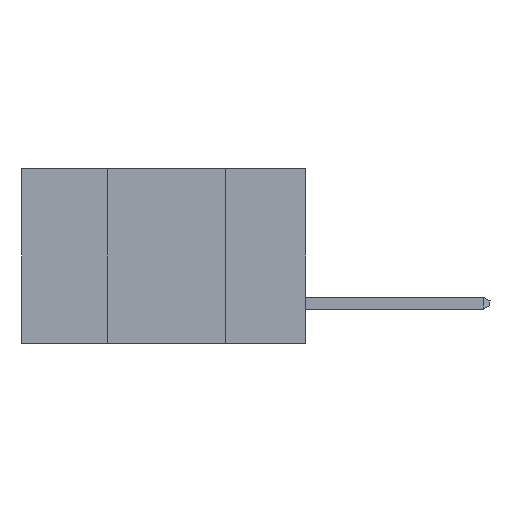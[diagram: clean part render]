
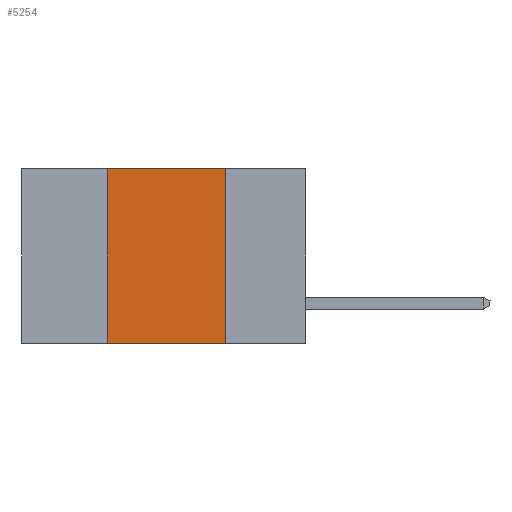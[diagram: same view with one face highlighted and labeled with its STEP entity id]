
A CAD part, left-side view. The second image highlights one B-rep face of the part: STEP entity #5254.
In plain terms, the highlighted planar face has unit normal (-1, 0, 0).
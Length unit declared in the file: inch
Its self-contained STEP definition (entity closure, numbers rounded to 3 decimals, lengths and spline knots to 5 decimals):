
#1218 = CARTESIAN_POINT ( 'NONE',  ( 0., 0.42, -0.37 ) ) ;
#2093 = ORIENTED_EDGE ( 'NONE', *, *, #2721, .F. ) ;
#2637 = CARTESIAN_POINT ( 'NONE',  ( 0., 0.17, -0.37 ) ) ;
#2721 = EDGE_CURVE ( 'NONE', #3608, #12944, #9174, .T. ) ;
#2815 = CARTESIAN_POINT ( 'NONE',  ( 0., 0.42, -0.37 ) ) ;
#2840 = VECTOR ( 'NONE', #8905, 39.37008 ) ;
#3608 = VERTEX_POINT ( 'NONE', #2815 ) ;
#3620 = PLANE ( 'NONE',  #11687 ) ;
#3855 = EDGE_CURVE ( 'NONE', #12944, #15523, #13419, .T. ) ;
#5254 = ADVANCED_FACE ( 'NONE', ( #11612 ), #3620, .F. ) ;
#5415 = CARTESIAN_POINT ( 'NONE',  ( 0., 0.6, 0. ) ) ;
#5866 = DIRECTION ( 'NONE',  ( 0., 0., -1. ) ) ;
#6260 = DIRECTION ( 'NONE',  ( 0., 0., -1. ) ) ;
#7070 = EDGE_LOOP ( 'NONE', ( #17733, #17338, #2093, #10352 ) ) ;
#7239 = CARTESIAN_POINT ( 'NONE',  ( 0., 0.17, -0.37 ) ) ;
#7947 = CARTESIAN_POINT ( 'NONE',  ( 0., 0.6, 0. ) ) ;
#8016 = VERTEX_POINT ( 'NONE', #2637 ) ;
#8419 = CARTESIAN_POINT ( 'NONE',  ( 0., 0.17, 0. ) ) ;
#8905 = DIRECTION ( 'NONE',  ( 0., -1., 0. ) ) ;
#8925 = VECTOR ( 'NONE', #19831, 39.37008 ) ;
#9110 = CARTESIAN_POINT ( 'NONE',  ( 0., 0.6, -0.37 ) ) ;
#9174 = LINE ( 'NONE', #1218, #18993 ) ;
#9486 = DIRECTION ( 'NONE',  ( 0., 0., 1. ) ) ;
#10352 = ORIENTED_EDGE ( 'NONE', *, *, #18750, .T. ) ;
#10399 = LINE ( 'NONE', #9110, #2840 ) ;
#11612 = FACE_OUTER_BOUND ( 'NONE', #7070, .T. ) ;
#11687 = AXIS2_PLACEMENT_3D ( 'NONE', #7947, #14856, #6260 ) ;
#12311 = LINE ( 'NONE', #7239, #19623 ) ;
#12944 = VERTEX_POINT ( 'NONE', #17665 ) ;
#13419 = LINE ( 'NONE', #5415, #8925 ) ;
#14856 = DIRECTION ( 'NONE',  ( 1., 0., 0. ) ) ;
#15523 = VERTEX_POINT ( 'NONE', #8419 ) ;
#17338 = ORIENTED_EDGE ( 'NONE', *, *, #3855, .F. ) ;
#17665 = CARTESIAN_POINT ( 'NONE',  ( 0., 0.42, 0. ) ) ;
#17733 = ORIENTED_EDGE ( 'NONE', *, *, #19963, .F. ) ;
#18750 = EDGE_CURVE ( 'NONE', #3608, #8016, #10399, .T. ) ;
#18993 = VECTOR ( 'NONE', #9486, 39.37008 ) ;
#19623 = VECTOR ( 'NONE', #5866, 39.37008 ) ;
#19831 = DIRECTION ( 'NONE',  ( 0., -1., 0. ) ) ;
#19963 = EDGE_CURVE ( 'NONE', #15523, #8016, #12311, .T. ) ;
